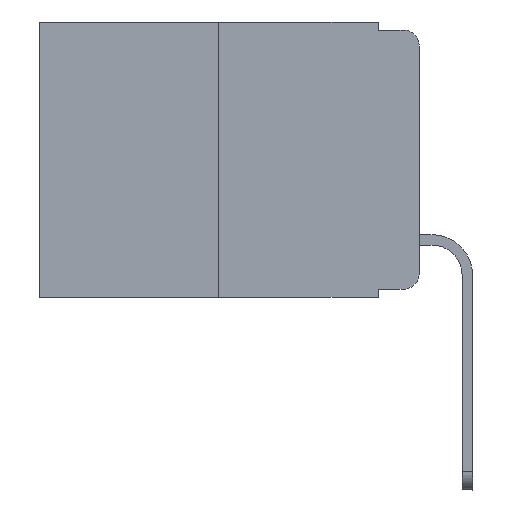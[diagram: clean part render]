
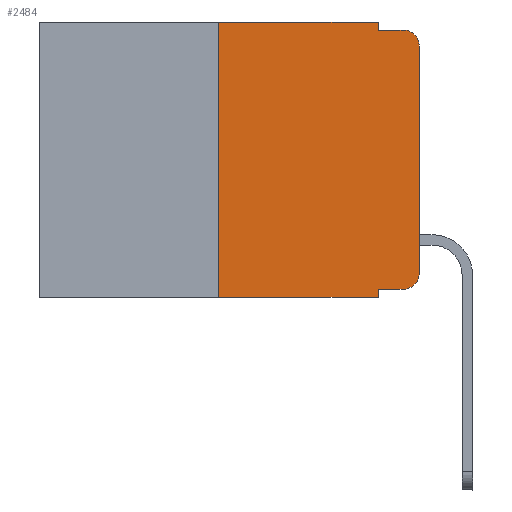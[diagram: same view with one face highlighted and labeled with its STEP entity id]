
A CAD part, left-side view. The second image highlights one B-rep face of the part: STEP entity #2484.
In plain terms, the highlighted planar face has unit normal (-1, 0, 0).
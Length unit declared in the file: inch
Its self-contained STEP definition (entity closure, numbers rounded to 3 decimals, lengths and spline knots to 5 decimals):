
#212 = VECTOR ( 'NONE', #277, 39.37008 ) ;
#277 = DIRECTION ( 'NONE',  ( 0., 0., -1. ) ) ;
#603 = DIRECTION ( 'NONE',  ( 0., -1., 0. ) ) ;
#689 = CIRCLE ( 'NONE', #8954, 0.02 ) ;
#710 = CARTESIAN_POINT ( 'NONE',  ( 0., 0.473, 0. ) ) ;
#818 = VECTOR ( 'NONE', #10036, 39.37008 ) ;
#822 = DIRECTION ( 'NONE',  ( 0., -1., 0. ) ) ;
#1149 = LINE ( 'NONE', #6606, #212 ) ;
#1176 = CARTESIAN_POINT ( 'NONE',  ( 0., 0., 0. ) ) ;
#1201 = DIRECTION ( 'NONE',  ( 0., 0., -1. ) ) ;
#1269 = CARTESIAN_POINT ( 'NONE',  ( 0., 0.051, 0. ) ) ;
#1609 = DIRECTION ( 'NONE',  ( 1., 0., 0. ) ) ;
#1790 = VERTEX_POINT ( 'NONE', #8397 ) ;
#2484 = ADVANCED_FACE ( 'NONE', ( #12233 ), #6947, .F. ) ;
#2741 = VERTEX_POINT ( 'NONE', #5663 ) ;
#2774 = CARTESIAN_POINT ( 'NONE',  ( 0., 0.051, -0.01 ) ) ;
#2956 = VECTOR ( 'NONE', #11389, 39.37008 ) ;
#2961 = EDGE_LOOP ( 'NONE', ( #13409, #10385, #3237, #7011, #8955, #11891, #13744, #7375, #8767, #7953 ) ) ;
#3071 = CARTESIAN_POINT ( 'NONE',  ( 0., 0.02, -0.01 ) ) ;
#3237 = ORIENTED_EDGE ( 'NONE', *, *, #6499, .F. ) ;
#3271 = EDGE_CURVE ( 'NONE', #11911, #12867, #9300, .T. ) ;
#3401 = LINE ( 'NONE', #1176, #7742 ) ;
#3446 = AXIS2_PLACEMENT_3D ( 'NONE', #12236, #12306, #4768 ) ;
#3496 = CARTESIAN_POINT ( 'NONE',  ( 0., 0.051, 0. ) ) ;
#3745 = LINE ( 'NONE', #2774, #6074 ) ;
#3985 = AXIS2_PLACEMENT_3D ( 'NONE', #710, #1609, #10141 ) ;
#4000 = EDGE_CURVE ( 'NONE', #1790, #7796, #689, .T. ) ;
#4058 = LINE ( 'NONE', #13326, #4976 ) ;
#4115 = EDGE_CURVE ( 'NONE', #9782, #7787, #1149, .T. ) ;
#4253 = CARTESIAN_POINT ( 'NONE',  ( 0., 0.473, -0.343 ) ) ;
#4329 = VERTEX_POINT ( 'NONE', #13567 ) ;
#4768 = DIRECTION ( 'NONE',  ( 0., 0., -1. ) ) ;
#4808 = CARTESIAN_POINT ( 'NONE',  ( 0., 0.25, 0. ) ) ;
#4976 = VECTOR ( 'NONE', #5110, 39.37008 ) ;
#5110 = DIRECTION ( 'NONE',  ( 0., -1., 0. ) ) ;
#5439 = EDGE_CURVE ( 'NONE', #11911, #2741, #9568, .T. ) ;
#5663 = CARTESIAN_POINT ( 'NONE',  ( 0., 0.051, -0.343 ) ) ;
#6024 = CARTESIAN_POINT ( 'NONE',  ( 0., 0.051, -0.333 ) ) ;
#6074 = VECTOR ( 'NONE', #603, 39.37008 ) ;
#6184 = EDGE_CURVE ( 'NONE', #12867, #9782, #4058, .T. ) ;
#6499 = EDGE_CURVE ( 'NONE', #7787, #7796, #3745, .T. ) ;
#6606 = CARTESIAN_POINT ( 'NONE',  ( 0., 0.051, 0. ) ) ;
#6672 = DIRECTION ( 'NONE',  ( 0., 0., -1. ) ) ;
#6770 = LINE ( 'NONE', #13299, #818 ) ;
#6947 = PLANE ( 'NONE',  #3985 ) ;
#7011 = ORIENTED_EDGE ( 'NONE', *, *, #4115, .F. ) ;
#7375 = ORIENTED_EDGE ( 'NONE', *, *, #10941, .F. ) ;
#7411 = CARTESIAN_POINT ( 'NONE',  ( 0., 0.02, -0.333 ) ) ;
#7677 = DIRECTION ( 'NONE',  ( 0., 0., 1. ) ) ;
#7742 = VECTOR ( 'NONE', #7677, 39.37008 ) ;
#7787 = VERTEX_POINT ( 'NONE', #8517 ) ;
#7796 = VERTEX_POINT ( 'NONE', #3071 ) ;
#7953 = ORIENTED_EDGE ( 'NONE', *, *, #9256, .T. ) ;
#8397 = CARTESIAN_POINT ( 'NONE',  ( 0., 0., -0.03 ) ) ;
#8500 = DIRECTION ( 'NONE',  ( -1., 0., 0. ) ) ;
#8517 = CARTESIAN_POINT ( 'NONE',  ( 0., 0.051, -0.01 ) ) ;
#8767 = ORIENTED_EDGE ( 'NONE', *, *, #13226, .T. ) ;
#8954 = AXIS2_PLACEMENT_3D ( 'NONE', #11716, #8500, #6672 ) ;
#8955 = ORIENTED_EDGE ( 'NONE', *, *, #6184, .F. ) ;
#9013 = VERTEX_POINT ( 'NONE', #6024 ) ;
#9256 = EDGE_CURVE ( 'NONE', #10575, #4329, #9269, .T. ) ;
#9269 = CIRCLE ( 'NONE', #3446, 0.02 ) ;
#9300 = LINE ( 'NONE', #4808, #2956 ) ;
#9568 = LINE ( 'NONE', #4253, #9864 ) ;
#9782 = VERTEX_POINT ( 'NONE', #3496 ) ;
#9812 = CARTESIAN_POINT ( 'NONE',  ( 0., 0.25, 0. ) ) ;
#9864 = VECTOR ( 'NONE', #822, 39.37008 ) ;
#10036 = DIRECTION ( 'NONE',  ( 0., -1., 0. ) ) ;
#10141 = DIRECTION ( 'NONE',  ( 0., 0., -1. ) ) ;
#10385 = ORIENTED_EDGE ( 'NONE', *, *, #4000, .T. ) ;
#10575 = VERTEX_POINT ( 'NONE', #7411 ) ;
#10941 = EDGE_CURVE ( 'NONE', #9013, #2741, #12931, .T. ) ;
#11389 = DIRECTION ( 'NONE',  ( 0., 0., 1. ) ) ;
#11716 = CARTESIAN_POINT ( 'NONE',  ( 0., 0.02, -0.03 ) ) ;
#11891 = ORIENTED_EDGE ( 'NONE', *, *, #3271, .F. ) ;
#11911 = VERTEX_POINT ( 'NONE', #12003 ) ;
#12003 = CARTESIAN_POINT ( 'NONE',  ( 0., 0.25, -0.343 ) ) ;
#12233 = FACE_OUTER_BOUND ( 'NONE', #2961, .T. ) ;
#12236 = CARTESIAN_POINT ( 'NONE',  ( 0., 0.02, -0.313 ) ) ;
#12306 = DIRECTION ( 'NONE',  ( -1., 0., 0. ) ) ;
#12867 = VERTEX_POINT ( 'NONE', #9812 ) ;
#12931 = LINE ( 'NONE', #1269, #13507 ) ;
#13095 = EDGE_CURVE ( 'NONE', #4329, #1790, #3401, .T. ) ;
#13226 = EDGE_CURVE ( 'NONE', #9013, #10575, #6770, .T. ) ;
#13299 = CARTESIAN_POINT ( 'NONE',  ( 0., 0.051, -0.333 ) ) ;
#13326 = CARTESIAN_POINT ( 'NONE',  ( 0., 0.473, 0. ) ) ;
#13409 = ORIENTED_EDGE ( 'NONE', *, *, #13095, .T. ) ;
#13507 = VECTOR ( 'NONE', #1201, 39.37008 ) ;
#13567 = CARTESIAN_POINT ( 'NONE',  ( 0., 0., -0.313 ) ) ;
#13744 = ORIENTED_EDGE ( 'NONE', *, *, #5439, .T. ) ;
